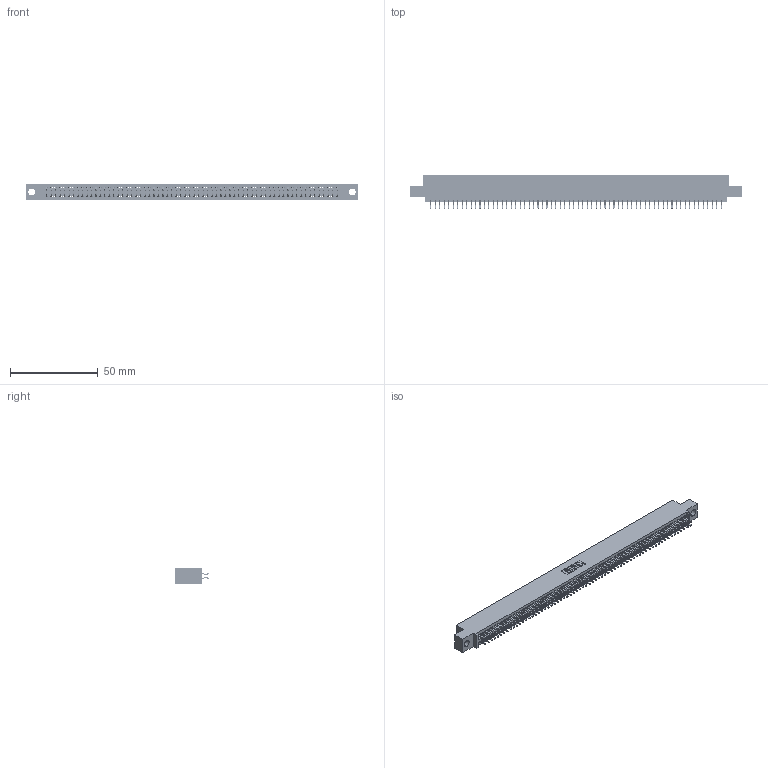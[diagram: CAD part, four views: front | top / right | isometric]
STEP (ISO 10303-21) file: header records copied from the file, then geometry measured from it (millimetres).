
FILE_DESCRIPTION (( 'STEP AP203' ), '1' );
FILE_NAME ('395-132-556-504.STEP', '2021-06-18T01:22:53', ( '' ), ( '' ), 'SwSTEP 2.0', 'SolidWorks 2020', '' );
FILE_SCHEMA (( 'CONFIG_CONTROL_DESIGN' ));
Length unit declared in the file: inch
Products named in the file (3): 345 Part_0.110 Offset - 0.156 Dia-TI; 395-132-556-504; 345-292-001_556 Tail
Assembly tree (133 placements, depth 2):
  395-132-556-504
    345 Part_0.110 Offset - 0.156 Dia-TI
    345-292-001_556 Tail  x132
Bounding box: 188.85 x 19.24 x 9.4 mm (x, y, z)
Volume: 18383.2 mm3; surface area: 27467.2 mm2
Topology: 133 solids, 133 shells, 7536 faces, 22433 edges, 14778 vertices
Faces by surface type: plane 4982, cylinder 2554
Entity records: 49325 total; most frequent: CARTESIAN_POINT 8266, ORIENTED_EDGE 8186, DIRECTION 7245, EDGE_CURVE 4093, VECTOR 3689, LINE 3689, VERTEX_POINT 2726, AXIS2_PLACEMENT_3D 1778
